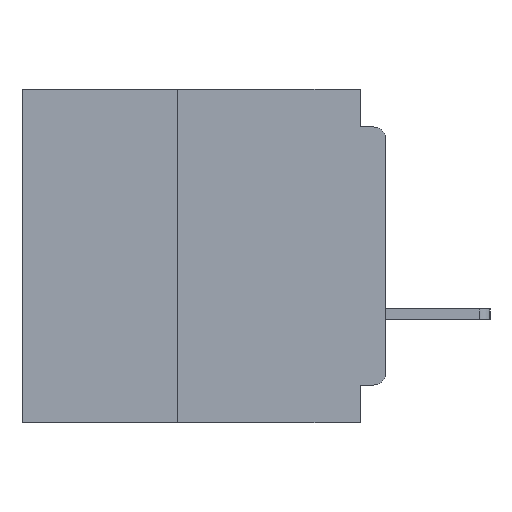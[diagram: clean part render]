
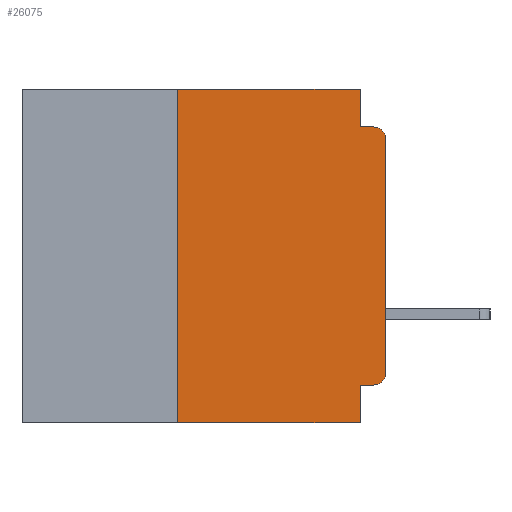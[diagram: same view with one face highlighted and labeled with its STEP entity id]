
A CAD part, left-side view. The second image highlights one B-rep face of the part: STEP entity #26075.
In plain terms, the highlighted planar face has unit normal (-1, 0, 0).
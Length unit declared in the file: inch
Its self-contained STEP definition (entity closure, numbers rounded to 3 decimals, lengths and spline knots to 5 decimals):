
#1093 = CARTESIAN_POINT ( 'NONE',  ( 0., 0.031, -0.355 ) ) ;
#2135 = DIRECTION ( 'NONE',  ( -1., 0., 0. ) ) ;
#2442 = LINE ( 'NONE', #45190, #22867 ) ;
#2762 = CARTESIAN_POINT ( 'NONE',  ( 0., 0.25, -0.4 ) ) ;
#3007 = VERTEX_POINT ( 'NONE', #28541 ) ;
#3899 = VECTOR ( 'NONE', #7465, 39.37008 ) ;
#4268 = VECTOR ( 'NONE', #40549, 39.37008 ) ;
#6493 = EDGE_CURVE ( 'NONE', #36509, #23511, #13804, .T. ) ;
#7047 = ORIENTED_EDGE ( 'NONE', *, *, #26242, .F. ) ;
#7120 = CARTESIAN_POINT ( 'NONE',  ( 0., 0.015, -0.355 ) ) ;
#7422 = LINE ( 'NONE', #32659, #27776 ) ;
#7465 = DIRECTION ( 'NONE',  ( 0., -1., 0. ) ) ;
#7940 = VERTEX_POINT ( 'NONE', #43454 ) ;
#8927 = CARTESIAN_POINT ( 'NONE',  ( 0., 0., -0.34 ) ) ;
#9633 = CARTESIAN_POINT ( 'NONE',  ( 0., 0.031, -0.045 ) ) ;
#10911 = DIRECTION ( 'NONE',  ( 0., -1., 0. ) ) ;
#11396 = EDGE_CURVE ( 'NONE', #30466, #3007, #44896, .T. ) ;
#11647 = LINE ( 'NONE', #43239, #12842 ) ;
#12842 = VECTOR ( 'NONE', #24304, 39.37008 ) ;
#13349 = AXIS2_PLACEMENT_3D ( 'NONE', #43103, #20354, #46889 ) ;
#13540 = EDGE_CURVE ( 'NONE', #7940, #47622, #36429, .T. ) ;
#13804 = LINE ( 'NONE', #15628, #23950 ) ;
#14139 = LINE ( 'NONE', #34248, #3899 ) ;
#14812 = CARTESIAN_POINT ( 'NONE',  ( 0., 0.015, -0.045 ) ) ;
#15514 = ORIENTED_EDGE ( 'NONE', *, *, #33874, .T. ) ;
#15517 = VERTEX_POINT ( 'NONE', #42031 ) ;
#15628 = CARTESIAN_POINT ( 'NONE',  ( 0., 0., 0. ) ) ;
#18238 = VERTEX_POINT ( 'NONE', #1093 ) ;
#18864 = FACE_OUTER_BOUND ( 'NONE', #44308, .T. ) ;
#19509 = ORIENTED_EDGE ( 'NONE', *, *, #47175, .F. ) ;
#20354 = DIRECTION ( 'NONE',  ( -1., 0., 0. ) ) ;
#20475 = VERTEX_POINT ( 'NONE', #14812 ) ;
#20709 = DIRECTION ( 'NONE',  ( 0., 0., -1. ) ) ;
#20824 = ORIENTED_EDGE ( 'NONE', *, *, #6493, .T. ) ;
#21210 = ORIENTED_EDGE ( 'NONE', *, *, #25343, .F. ) ;
#22867 = VECTOR ( 'NONE', #10911, 39.37008 ) ;
#23511 = VERTEX_POINT ( 'NONE', #31965 ) ;
#23950 = VECTOR ( 'NONE', #42267, 39.37008 ) ;
#24304 = DIRECTION ( 'NONE',  ( 0., 1., 0. ) ) ;
#24650 = LINE ( 'NONE', #48115, #4268 ) ;
#25095 = CARTESIAN_POINT ( 'NONE',  ( 0., 0.015, -0.06 ) ) ;
#25343 = EDGE_CURVE ( 'NONE', #3007, #7940, #14139, .T. ) ;
#26075 = ADVANCED_FACE ( 'NONE', ( #18864 ), #38486, .F. ) ;
#26242 = EDGE_CURVE ( 'NONE', #28781, #18238, #11647, .T. ) ;
#26970 = DIRECTION ( 'NONE',  ( 1., 0., 0. ) ) ;
#27573 = ORIENTED_EDGE ( 'NONE', *, *, #13540, .F. ) ;
#27776 = VECTOR ( 'NONE', #43917, 39.37008 ) ;
#28541 = CARTESIAN_POINT ( 'NONE',  ( 0., 0.25, 0. ) ) ;
#28781 = VERTEX_POINT ( 'NONE', #7120 ) ;
#28947 = DIRECTION ( 'NONE',  ( 0., 0., -1. ) ) ;
#30046 = EDGE_CURVE ( 'NONE', #30466, #15517, #2442, .T. ) ;
#30072 = ORIENTED_EDGE ( 'NONE', *, *, #30046, .T. ) ;
#30466 = VERTEX_POINT ( 'NONE', #32741 ) ;
#31397 = CIRCLE ( 'NONE', #40772, 0.015 ) ;
#31460 = ORIENTED_EDGE ( 'NONE', *, *, #43253, .T. ) ;
#31965 = CARTESIAN_POINT ( 'NONE',  ( 0., 0., -0.06 ) ) ;
#32659 = CARTESIAN_POINT ( 'NONE',  ( 0., 0., -0.045 ) ) ;
#32741 = CARTESIAN_POINT ( 'NONE',  ( 0., 0.25, -0.4 ) ) ;
#33414 = DIRECTION ( 'NONE',  ( 0., 0., 1. ) ) ;
#33874 = EDGE_CURVE ( 'NONE', #23511, #20475, #31397, .T. ) ;
#34047 = VECTOR ( 'NONE', #20709, 39.37008 ) ;
#34248 = CARTESIAN_POINT ( 'NONE',  ( 0., 0.437, 0. ) ) ;
#34669 = CARTESIAN_POINT ( 'NONE',  ( 0., 0.437, 0. ) ) ;
#36429 = LINE ( 'NONE', #47230, #34047 ) ;
#36509 = VERTEX_POINT ( 'NONE', #8927 ) ;
#38486 = PLANE ( 'NONE',  #45903 ) ;
#39358 = EDGE_CURVE ( 'NONE', #18238, #15517, #24650, .T. ) ;
#39699 = CIRCLE ( 'NONE', #13349, 0.015 ) ;
#40549 = DIRECTION ( 'NONE',  ( 0., 0., -1. ) ) ;
#40772 = AXIS2_PLACEMENT_3D ( 'NONE', #25095, #2135, #28947 ) ;
#42031 = CARTESIAN_POINT ( 'NONE',  ( 0., 0.031, -0.4 ) ) ;
#42267 = DIRECTION ( 'NONE',  ( 0., 0., 1. ) ) ;
#42272 = DIRECTION ( 'NONE',  ( 0., 0., -1. ) ) ;
#43103 = CARTESIAN_POINT ( 'NONE',  ( 0., 0.015, -0.34 ) ) ;
#43239 = CARTESIAN_POINT ( 'NONE',  ( 0., 0., -0.355 ) ) ;
#43253 = EDGE_CURVE ( 'NONE', #28781, #36509, #39699, .T. ) ;
#43322 = ORIENTED_EDGE ( 'NONE', *, *, #39358, .F. ) ;
#43454 = CARTESIAN_POINT ( 'NONE',  ( 0., 0.031, 0. ) ) ;
#43715 = VECTOR ( 'NONE', #33414, 39.37008 ) ;
#43917 = DIRECTION ( 'NONE',  ( 0., -1., 0. ) ) ;
#44040 = ORIENTED_EDGE ( 'NONE', *, *, #11396, .F. ) ;
#44308 = EDGE_LOOP ( 'NONE', ( #20824, #15514, #19509, #27573, #21210, #44040, #30072, #43322, #7047, #31460 ) ) ;
#44896 = LINE ( 'NONE', #2762, #43715 ) ;
#45190 = CARTESIAN_POINT ( 'NONE',  ( 0., 0.437, -0.4 ) ) ;
#45903 = AXIS2_PLACEMENT_3D ( 'NONE', #34669, #26970, #42272 ) ;
#46889 = DIRECTION ( 'NONE',  ( 0., 0., -1. ) ) ;
#47175 = EDGE_CURVE ( 'NONE', #47622, #20475, #7422, .T. ) ;
#47230 = CARTESIAN_POINT ( 'NONE',  ( 0., 0.031, 0. ) ) ;
#47622 = VERTEX_POINT ( 'NONE', #9633 ) ;
#48115 = CARTESIAN_POINT ( 'NONE',  ( 0., 0.031, -0.4 ) ) ;
